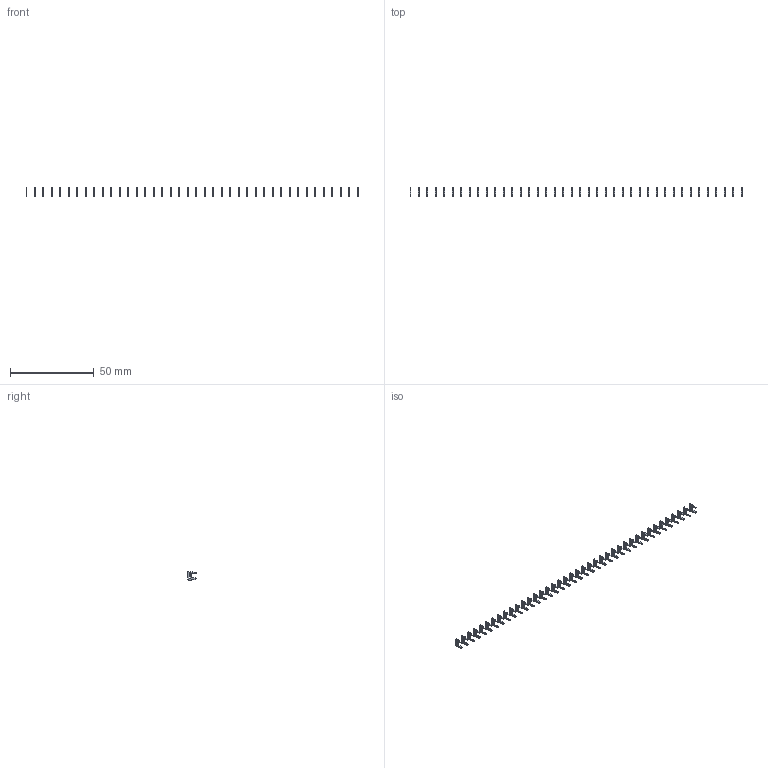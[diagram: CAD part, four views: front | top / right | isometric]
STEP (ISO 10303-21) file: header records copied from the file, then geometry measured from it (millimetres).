
FILE_DESCRIPTION (( 'STEP AP203' ), '1' );
FILE_NAME ('105-040-208-200.STEP', '2020-04-07T23:57:42', ( '' ), ( '' ), 'SwSTEP 2.0', 'SolidWorks 2016', '' );
FILE_SCHEMA (( 'CONFIG_CONTROL_DESIGN' ));
Length unit declared in the file: inch
Products named in the file (2): 105-040-208-200; 100-290-001_100-290-208
Assembly tree (40 placements, depth 2):
  105-040-208-200
    100-290-001_100-290-208  x40
Bounding box: 198.63 x 4.83 x 5.17 mm (x, y, z)
Volume: 275.2 mm3; surface area: 1699.8 mm2
Topology: 40 solids, 40 shells, 1000 faces, 2760 edges, 1840 vertices
Faces by surface type: plane 880, cylinder 120
Entity records: 2237 total; most frequent: DIRECTION 211, CARTESIAN_POINT 183, ORIENTED_EDGE 138, LOCAL_TIME 90, COORDINATED_UNIVERSAL_TIME_OFFSET 90, CALENDAR_DATE 90, DATE_AND_TIME 90, AXIS2_PLACEMENT_3D 74
